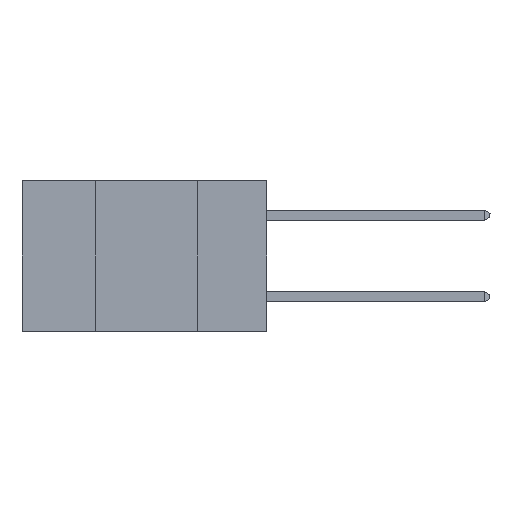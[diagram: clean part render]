
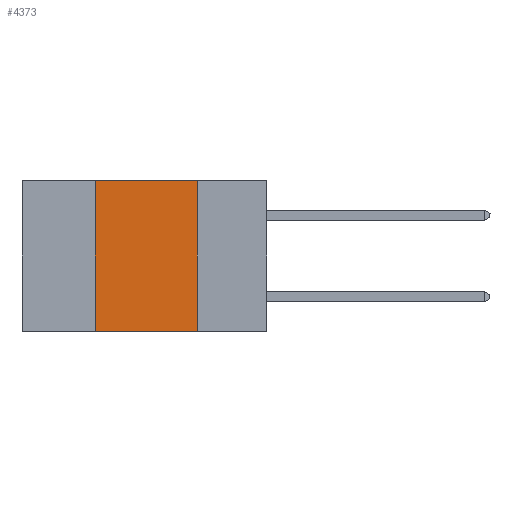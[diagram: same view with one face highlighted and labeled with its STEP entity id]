
A CAD part, left-side view. The second image highlights one B-rep face of the part: STEP entity #4373.
In plain terms, the highlighted planar face has unit normal (-1, 0, 0).
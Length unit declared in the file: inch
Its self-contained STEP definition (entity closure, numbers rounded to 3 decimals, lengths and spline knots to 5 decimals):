
#429 = CARTESIAN_POINT ( 'NONE',  ( 0., 0.6, 0. ) ) ;
#1055 = EDGE_CURVE ( 'NONE', #3751, #8412, #15698, .T. ) ;
#1153 = LINE ( 'NONE', #14028, #14041 ) ;
#1204 = FACE_OUTER_BOUND ( 'NONE', #13294, .T. ) ;
#1250 = LINE ( 'NONE', #2879, #7654 ) ;
#2605 = ORIENTED_EDGE ( 'NONE', *, *, #1055, .T. ) ;
#2879 = CARTESIAN_POINT ( 'NONE',  ( 0., 0.42, 0. ) ) ;
#3751 = VERTEX_POINT ( 'NONE', #7457 ) ;
#4320 = CARTESIAN_POINT ( 'NONE',  ( 0., 0.42, 0. ) ) ;
#4373 = ADVANCED_FACE ( 'NONE', ( #1204 ), #8705, .F. ) ;
#4605 = EDGE_CURVE ( 'NONE', #3751, #12782, #1250, .T. ) ;
#6057 = ORIENTED_EDGE ( 'NONE', *, *, #4605, .F. ) ;
#6322 = ORIENTED_EDGE ( 'NONE', *, *, #19416, .F. ) ;
#7411 = DIRECTION ( 'NONE',  ( 0., 0., 1. ) ) ;
#7457 = CARTESIAN_POINT ( 'NONE',  ( 0., 0.42, -0.37 ) ) ;
#7654 = VECTOR ( 'NONE', #7411, 39.37008 ) ;
#8412 = VERTEX_POINT ( 'NONE', #16526 ) ;
#8604 = VECTOR ( 'NONE', #9534, 39.37008 ) ;
#8705 = PLANE ( 'NONE',  #9713 ) ;
#9534 = DIRECTION ( 'NONE',  ( 0., 0., -1. ) ) ;
#9713 = AXIS2_PLACEMENT_3D ( 'NONE', #429, #18427, #18100 ) ;
#10842 = LINE ( 'NONE', #10938, #8604 ) ;
#10917 = CARTESIAN_POINT ( 'NONE',  ( 0., 0.6, -0.37 ) ) ;
#10938 = CARTESIAN_POINT ( 'NONE',  ( 0., 0.17, 0. ) ) ;
#11105 = ORIENTED_EDGE ( 'NONE', *, *, #16477, .F. ) ;
#12782 = VERTEX_POINT ( 'NONE', #4320 ) ;
#13294 = EDGE_LOOP ( 'NONE', ( #6322, #11105, #6057, #2605 ) ) ;
#14028 = CARTESIAN_POINT ( 'NONE',  ( 0., 0.6, 0. ) ) ;
#14041 = VECTOR ( 'NONE', #17558, 39.37008 ) ;
#15698 = LINE ( 'NONE', #10917, #19194 ) ;
#16477 = EDGE_CURVE ( 'NONE', #12782, #18239, #1153, .T. ) ;
#16526 = CARTESIAN_POINT ( 'NONE',  ( 0., 0.17, -0.37 ) ) ;
#17558 = DIRECTION ( 'NONE',  ( 0., -1., 0. ) ) ;
#17640 = CARTESIAN_POINT ( 'NONE',  ( 0., 0.17, 0. ) ) ;
#18100 = DIRECTION ( 'NONE',  ( 0., 0., -1. ) ) ;
#18239 = VERTEX_POINT ( 'NONE', #17640 ) ;
#18427 = DIRECTION ( 'NONE',  ( 1., 0., 0. ) ) ;
#18911 = DIRECTION ( 'NONE',  ( 0., -1., 0. ) ) ;
#19194 = VECTOR ( 'NONE', #18911, 39.37008 ) ;
#19416 = EDGE_CURVE ( 'NONE', #18239, #8412, #10842, .T. ) ;
